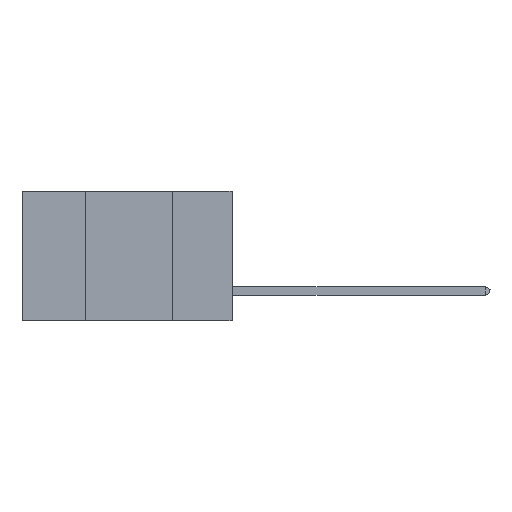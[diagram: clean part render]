
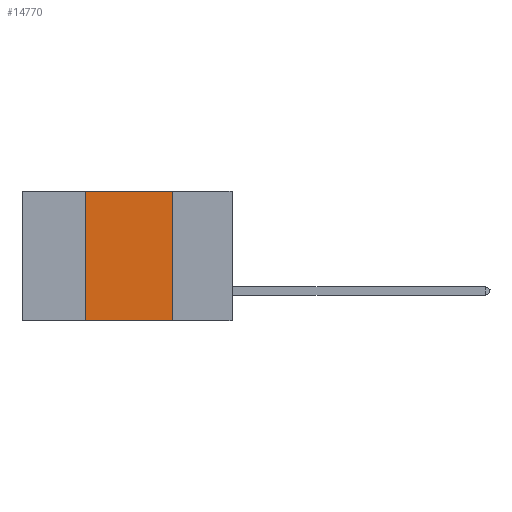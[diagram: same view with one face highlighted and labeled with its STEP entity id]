
A CAD part, left-side view. The second image highlights one B-rep face of the part: STEP entity #14770.
In plain terms, the highlighted planar face has unit normal (-1, 0, 0).
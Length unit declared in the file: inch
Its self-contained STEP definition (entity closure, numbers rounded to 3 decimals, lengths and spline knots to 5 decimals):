
#755 = VERTEX_POINT ( 'NONE', #4159 ) ;
#883 = LINE ( 'NONE', #10390, #13577 ) ;
#2650 = DIRECTION ( 'NONE',  ( 0., -1., 0. ) ) ;
#2936 = ORIENTED_EDGE ( 'NONE', *, *, #17476, .F. ) ;
#3645 = ORIENTED_EDGE ( 'NONE', *, *, #39997, .F. ) ;
#4159 = CARTESIAN_POINT ( 'NONE',  ( 0., 0.17, 0. ) ) ;
#4291 = DIRECTION ( 'NONE',  ( 1., 0., 0. ) ) ;
#9463 = VERTEX_POINT ( 'NONE', #17557 ) ;
#9509 = DIRECTION ( 'NONE',  ( 0., -1., 0. ) ) ;
#10390 = CARTESIAN_POINT ( 'NONE',  ( 0., 0.17, 0. ) ) ;
#12897 = CARTESIAN_POINT ( 'NONE',  ( 0., 0.6, 0. ) ) ;
#13577 = VECTOR ( 'NONE', #36524, 39.37008 ) ;
#14770 = ADVANCED_FACE ( 'NONE', ( #38926 ), #16960, .F. ) ;
#15971 = EDGE_CURVE ( 'NONE', #38591, #9463, #35653, .T. ) ;
#16280 = EDGE_CURVE ( 'NONE', #38591, #19497, #33190, .T. ) ;
#16960 = PLANE ( 'NONE',  #30941 ) ;
#17313 = CARTESIAN_POINT ( 'NONE',  ( 0., 0.42, 0. ) ) ;
#17476 = EDGE_CURVE ( 'NONE', #755, #19497, #883, .T. ) ;
#17557 = CARTESIAN_POINT ( 'NONE',  ( 0., 0.42, 0. ) ) ;
#18391 = EDGE_LOOP ( 'NONE', ( #2936, #3645, #31810, #27568 ) ) ;
#19497 = VERTEX_POINT ( 'NONE', #21423 ) ;
#20250 = VECTOR ( 'NONE', #9509, 39.37008 ) ;
#21423 = CARTESIAN_POINT ( 'NONE',  ( 0., 0.17, -0.37 ) ) ;
#22458 = VECTOR ( 'NONE', #2650, 39.37008 ) ;
#23173 = DIRECTION ( 'NONE',  ( 0., 0., -1. ) ) ;
#23401 = DIRECTION ( 'NONE',  ( 0., 0., 1. ) ) ;
#26891 = VECTOR ( 'NONE', #23401, 39.37008 ) ;
#27568 = ORIENTED_EDGE ( 'NONE', *, *, #16280, .T. ) ;
#27752 = CARTESIAN_POINT ( 'NONE',  ( 0., 0.6, -0.37 ) ) ;
#28090 = CARTESIAN_POINT ( 'NONE',  ( 0., 0.42, -0.37 ) ) ;
#30941 = AXIS2_PLACEMENT_3D ( 'NONE', #38755, #4291, #23173 ) ;
#31810 = ORIENTED_EDGE ( 'NONE', *, *, #15971, .F. ) ;
#33190 = LINE ( 'NONE', #27752, #22458 ) ;
#35653 = LINE ( 'NONE', #17313, #26891 ) ;
#36524 = DIRECTION ( 'NONE',  ( 0., 0., -1. ) ) ;
#37866 = LINE ( 'NONE', #12897, #20250 ) ;
#38591 = VERTEX_POINT ( 'NONE', #28090 ) ;
#38755 = CARTESIAN_POINT ( 'NONE',  ( 0., 0.6, 0. ) ) ;
#38926 = FACE_OUTER_BOUND ( 'NONE', #18391, .T. ) ;
#39997 = EDGE_CURVE ( 'NONE', #9463, #755, #37866, .T. ) ;
